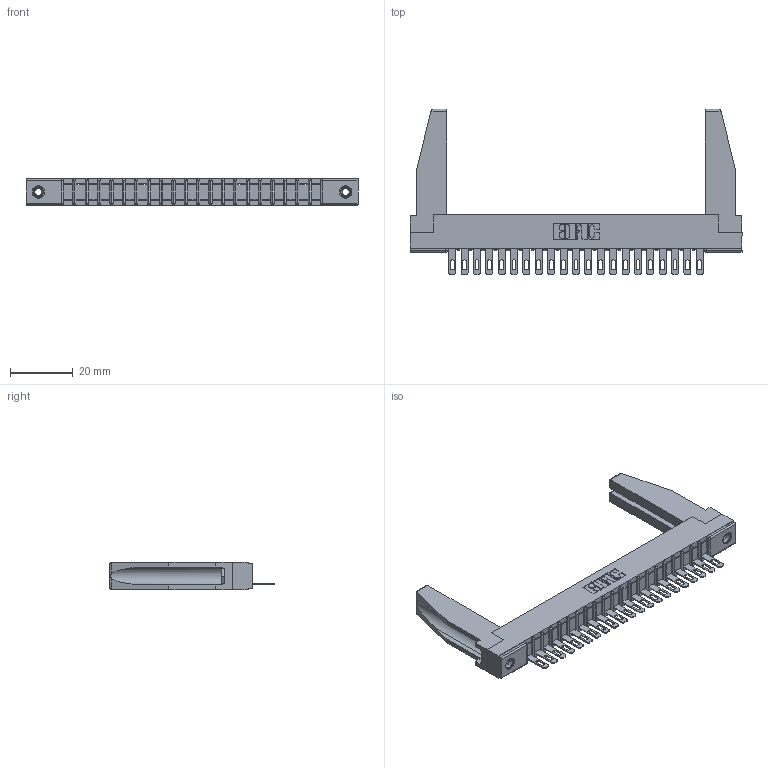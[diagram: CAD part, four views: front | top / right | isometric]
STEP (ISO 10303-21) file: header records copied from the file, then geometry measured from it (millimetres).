
FILE_DESCRIPTION (( 'STEP AP203' ), '1' );
FILE_NAME ('357-021-505-178.STEP', '2019-09-13T23:23:52', ( '' ), ( '' ), 'SwSTEP 2.0', 'SolidWorks 2016', '' );
FILE_SCHEMA (( 'CONFIG_CONTROL_DESIGN' ));
Length unit declared in the file: inch
Products named in the file (5): 357-021-505-178; 307 Part_.156 Dia Mounting Holes; 307-220-078; 345-250-001_345-250-001-102; 307-290-001_505
Assembly tree (26 placements, depth 2):
  357-021-505-178
    307 Part_.156 Dia Mounting Holes
    307-290-001_505  x21
    307-220-078  x2
    345-250-001_345-250-001-102  x2
Bounding box: 106.22 x 52.88 x 8.71 mm (x, y, z)
Volume: 10730.8 mm3; surface area: 14406.3 mm2
Topology: 26 solids, 26 shells, 1446 faces, 4055 edges, 2606 vertices
Faces by surface type: plane 910, cylinder 476, sphere 44, cone 12, torus 4
Entity records: 23005 total; most frequent: CARTESIAN_POINT 3866, ORIENTED_EDGE 3808, DIRECTION 3730, EDGE_CURVE 1904, LINE 1454, VECTOR 1454, VERTEX_POINT 1232, AXIS2_PLACEMENT_3D 1138
